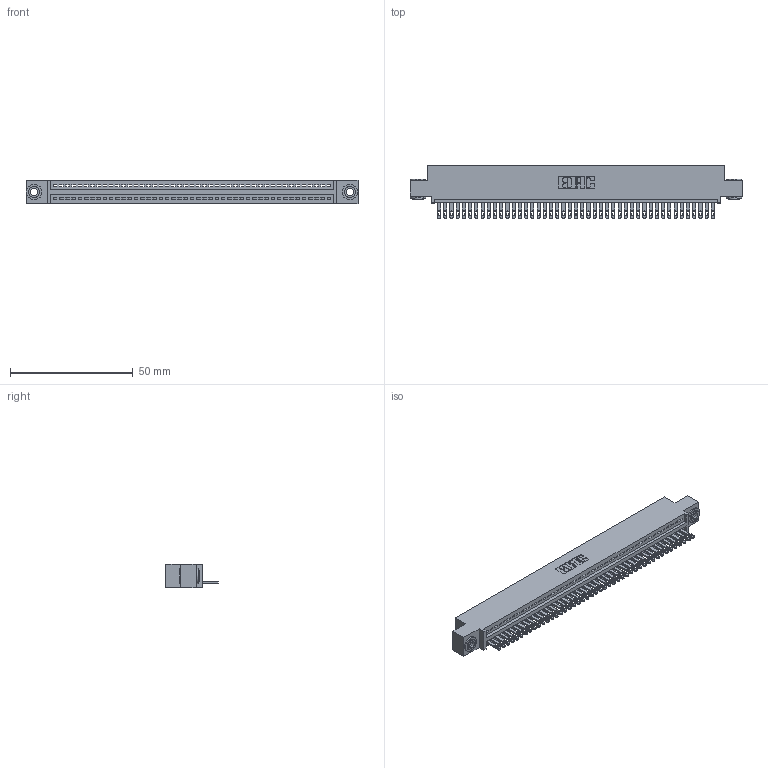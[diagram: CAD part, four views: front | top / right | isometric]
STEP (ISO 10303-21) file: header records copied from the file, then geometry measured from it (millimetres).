
FILE_DESCRIPTION (( 'STEP AP203' ), '1' );
FILE_NAME ('895-045-500-403.STEP', '2020-09-27T04:00:37', ( '' ), ( '' ), 'SwSTEP 2.0', 'SolidWorks 2020', '' );
FILE_SCHEMA (( 'CONFIG_CONTROL_DESIGN' ));
Length unit declared in the file: inch
Products named in the file (4): 345-292-001_345-293-100; 845 Part_0.110 Offset - 0.156 Dia-TH; 895-045-500-403; 345-250-002_345-250-002-102
Assembly tree (48 placements, depth 2):
  895-045-500-403
    845 Part_0.110 Offset - 0.156 Dia-TH
    345-292-001_345-293-100  x45
    345-250-002_345-250-002-102  x2
Bounding box: 135.51 x 21.51 x 9.4 mm (x, y, z)
Volume: 12869.2 mm3; surface area: 17540.3 mm2
Topology: 48 solids, 48 shells, 2598 faces, 7989 edges, 5322 vertices
Faces by surface type: plane 1624, cylinder 966, cone 8
Entity records: 34176 total; most frequent: CARTESIAN_POINT 5898, ORIENTED_EDGE 5870, DIRECTION 5179, EDGE_CURVE 2935, LINE 2595, VECTOR 2595, VERTEX_POINT 1954, AXIS2_PLACEMENT_3D 1292
